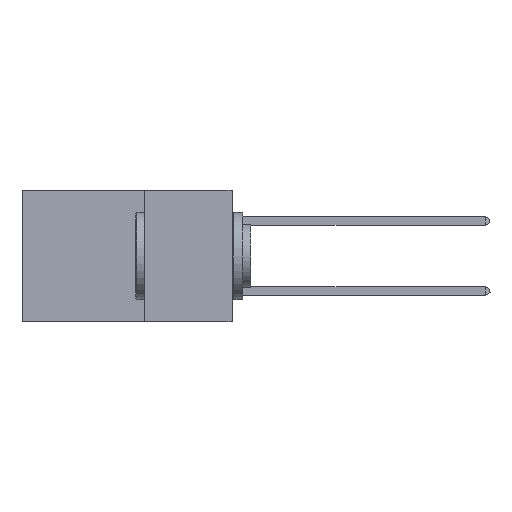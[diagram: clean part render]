
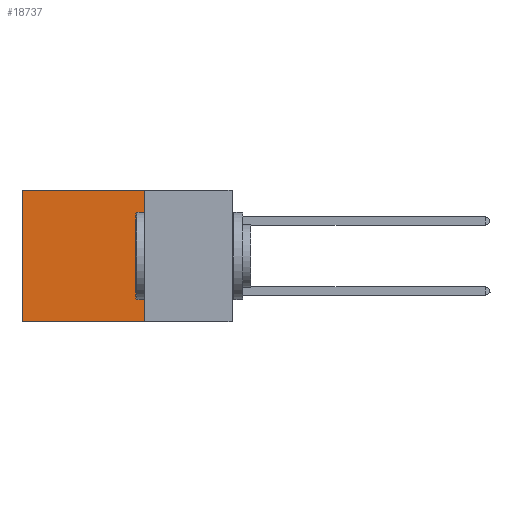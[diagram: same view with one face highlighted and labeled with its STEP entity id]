
A CAD part, left-side view. The second image highlights one B-rep face of the part: STEP entity #18737.
In plain terms, the highlighted planar face has unit normal (-1, 0, 0).
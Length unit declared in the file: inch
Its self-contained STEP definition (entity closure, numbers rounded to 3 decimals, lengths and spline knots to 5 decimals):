
#200 = CARTESIAN_POINT ( 'NONE',  ( 0.2875, 0.6, -0.375 ) ) ;
#890 = VECTOR ( 'NONE', #8770, 39.37008 ) ;
#1434 = EDGE_CURVE ( 'NONE', #3280, #10306, #13974, .T. ) ;
#3280 = VERTEX_POINT ( 'NONE', #8396 ) ;
#3359 = CARTESIAN_POINT ( 'NONE',  ( 0.2875, 0.25, 0. ) ) ;
#3486 = DIRECTION ( 'NONE',  ( 0., 1., 0. ) ) ;
#3733 = VERTEX_POINT ( 'NONE', #200 ) ;
#5272 = VERTEX_POINT ( 'NONE', #16484 ) ;
#5834 = ORIENTED_EDGE ( 'NONE', *, *, #1434, .T. ) ;
#6336 = CARTESIAN_POINT ( 'NONE',  ( 0.2875, 0.25, -0.375 ) ) ;
#6712 = PLANE ( 'NONE',  #10867 ) ;
#7260 = CARTESIAN_POINT ( 'NONE',  ( 0.2875, 0.6, -0.375 ) ) ;
#7423 = CARTESIAN_POINT ( 'NONE',  ( 0.2875, 0.25, -0.375 ) ) ;
#7691 = ORIENTED_EDGE ( 'NONE', *, *, #18666, .F. ) ;
#8076 = ORIENTED_EDGE ( 'NONE', *, *, #17396, .T. ) ;
#8140 = DIRECTION ( 'NONE',  ( 1., 0., 0. ) ) ;
#8396 = CARTESIAN_POINT ( 'NONE',  ( 0.2875, 0.25, 0. ) ) ;
#8770 = DIRECTION ( 'NONE',  ( 0., 0., -1. ) ) ;
#8840 = LINE ( 'NONE', #7260, #890 ) ;
#10306 = VERTEX_POINT ( 'NONE', #14092 ) ;
#10411 = DIRECTION ( 'NONE',  ( 0., 1., 0. ) ) ;
#10616 = LINE ( 'NONE', #7423, #16891 ) ;
#10837 = FACE_OUTER_BOUND ( 'NONE', #16863, .T. ) ;
#10867 = AXIS2_PLACEMENT_3D ( 'NONE', #15607, #8140, #12608 ) ;
#12608 = DIRECTION ( 'NONE',  ( 0., 0., -1. ) ) ;
#13974 = LINE ( 'NONE', #3359, #16288 ) ;
#14092 = CARTESIAN_POINT ( 'NONE',  ( 0.2875, 0.6, 0. ) ) ;
#15145 = DIRECTION ( 'NONE',  ( 0., 0., -1. ) ) ;
#15258 = VECTOR ( 'NONE', #15145, 39.37008 ) ;
#15607 = CARTESIAN_POINT ( 'NONE',  ( 0.2875, 0.25, -0.375 ) ) ;
#16288 = VECTOR ( 'NONE', #3486, 39.37008 ) ;
#16484 = CARTESIAN_POINT ( 'NONE',  ( 0.2875, 0.25, -0.375 ) ) ;
#16652 = LINE ( 'NONE', #6336, #15258 ) ;
#16863 = EDGE_LOOP ( 'NONE', ( #8076, #18414, #7691, #5834 ) ) ;
#16891 = VECTOR ( 'NONE', #10411, 39.37008 ) ;
#17396 = EDGE_CURVE ( 'NONE', #10306, #3733, #8840, .T. ) ;
#18414 = ORIENTED_EDGE ( 'NONE', *, *, #18572, .F. ) ;
#18572 = EDGE_CURVE ( 'NONE', #5272, #3733, #10616, .T. ) ;
#18666 = EDGE_CURVE ( 'NONE', #3280, #5272, #16652, .T. ) ;
#18737 = ADVANCED_FACE ( 'NONE', ( #10837 ), #6712, .F. ) ;
